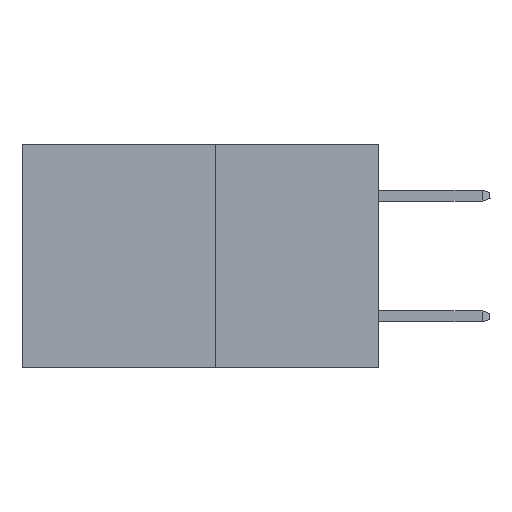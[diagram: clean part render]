
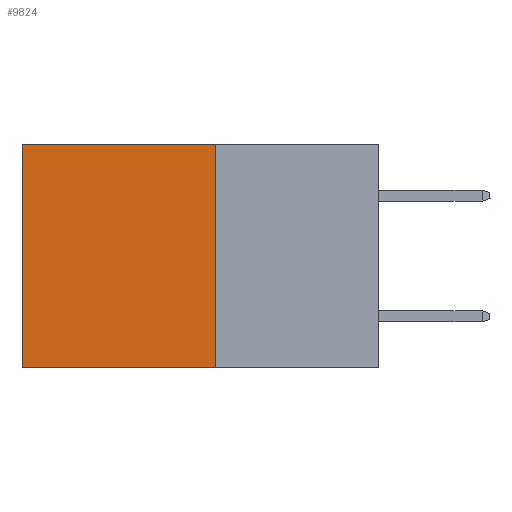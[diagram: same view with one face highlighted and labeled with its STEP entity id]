
A CAD part, left-side view. The second image highlights one B-rep face of the part: STEP entity #9824.
In plain terms, the highlighted planar face has unit normal (-1, 0, 0).
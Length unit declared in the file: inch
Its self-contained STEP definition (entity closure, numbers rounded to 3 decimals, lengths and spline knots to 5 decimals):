
#522 = DIRECTION ( 'NONE',  ( 0., 0., -1. ) ) ;
#622 = DIRECTION ( 'NONE',  ( 0., 0., -1. ) ) ;
#746 = VECTOR ( 'NONE', #522, 39.37008 ) ;
#874 = EDGE_LOOP ( 'NONE', ( #5247, #1437, #2615, #3825 ) ) ;
#966 = DIRECTION ( 'NONE',  ( 0., 1., 0. ) ) ;
#1154 = VERTEX_POINT ( 'NONE', #4227 ) ;
#1437 = ORIENTED_EDGE ( 'NONE', *, *, #2765, .F. ) ;
#2230 = CARTESIAN_POINT ( 'NONE',  ( 0.277, 0.59, -0.37 ) ) ;
#2322 = CARTESIAN_POINT ( 'NONE',  ( 0.277, 0.27, -0.37 ) ) ;
#2358 = CARTESIAN_POINT ( 'NONE',  ( 0.277, 0.27, -0.37 ) ) ;
#2615 = ORIENTED_EDGE ( 'NONE', *, *, #3591, .F. ) ;
#2765 = EDGE_CURVE ( 'NONE', #6982, #4105, #8945, .T. ) ;
#3050 = VECTOR ( 'NONE', #6364, 39.37008 ) ;
#3423 = CARTESIAN_POINT ( 'NONE',  ( 0.277, 0.27, 0. ) ) ;
#3591 = EDGE_CURVE ( 'NONE', #1154, #6982, #10039, .T. ) ;
#3664 = VERTEX_POINT ( 'NONE', #4625 ) ;
#3825 = ORIENTED_EDGE ( 'NONE', *, *, #9505, .T. ) ;
#3941 = DIRECTION ( 'NONE',  ( 0., 0., -1. ) ) ;
#4105 = VERTEX_POINT ( 'NONE', #5190 ) ;
#4227 = CARTESIAN_POINT ( 'NONE',  ( 0.277, 0.27, 0. ) ) ;
#4555 = CARTESIAN_POINT ( 'NONE',  ( 0.277, 0.27, -0.37 ) ) ;
#4625 = CARTESIAN_POINT ( 'NONE',  ( 0.277, 0.59, 0. ) ) ;
#4901 = FACE_OUTER_BOUND ( 'NONE', #874, .T. ) ;
#5146 = AXIS2_PLACEMENT_3D ( 'NONE', #2322, #8519, #3941 ) ;
#5190 = CARTESIAN_POINT ( 'NONE',  ( 0.277, 0.59, -0.37 ) ) ;
#5247 = ORIENTED_EDGE ( 'NONE', *, *, #6907, .T. ) ;
#6364 = DIRECTION ( 'NONE',  ( 0., 1., 0. ) ) ;
#6518 = CARTESIAN_POINT ( 'NONE',  ( 0.277, 0.27, -0.37 ) ) ;
#6907 = EDGE_CURVE ( 'NONE', #3664, #4105, #8827, .T. ) ;
#6920 = VECTOR ( 'NONE', #622, 39.37008 ) ;
#6982 = VERTEX_POINT ( 'NONE', #2358 ) ;
#7783 = VECTOR ( 'NONE', #966, 39.37008 ) ;
#7815 = PLANE ( 'NONE',  #5146 ) ;
#8519 = DIRECTION ( 'NONE',  ( 1., 0., 0. ) ) ;
#8827 = LINE ( 'NONE', #2230, #6920 ) ;
#8945 = LINE ( 'NONE', #6518, #3050 ) ;
#9505 = EDGE_CURVE ( 'NONE', #1154, #3664, #9904, .T. ) ;
#9824 = ADVANCED_FACE ( 'NONE', ( #4901 ), #7815, .F. ) ;
#9904 = LINE ( 'NONE', #3423, #7783 ) ;
#10039 = LINE ( 'NONE', #4555, #746 ) ;
